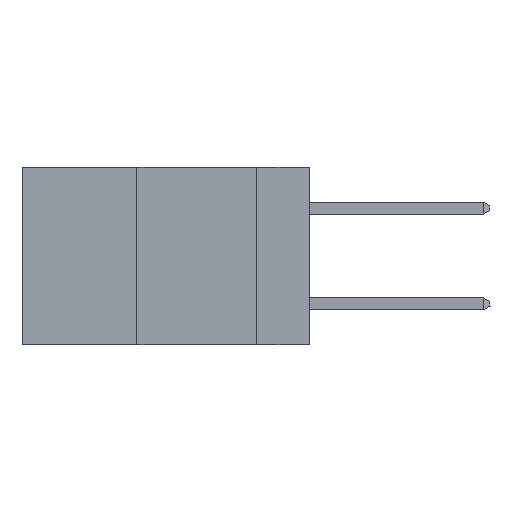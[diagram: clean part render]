
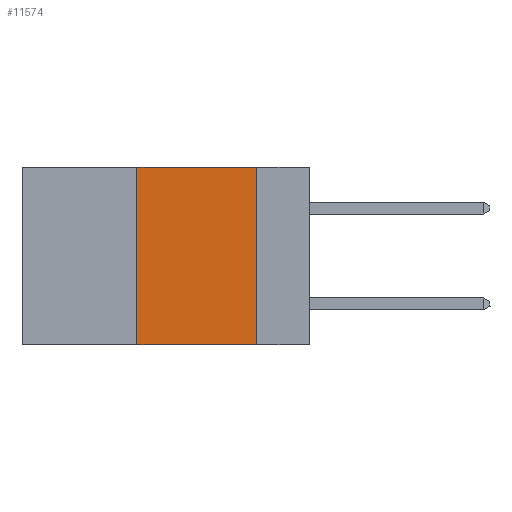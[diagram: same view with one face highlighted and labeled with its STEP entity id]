
A CAD part, left-side view. The second image highlights one B-rep face of the part: STEP entity #11574.
In plain terms, the highlighted planar face has unit normal (-1, 0, 0).
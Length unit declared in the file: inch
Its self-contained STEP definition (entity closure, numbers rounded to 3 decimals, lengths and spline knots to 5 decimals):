
#11 = CARTESIAN_POINT ( 'NONE',  ( 0., 0.11, 0. ) ) ;
#1041 = LINE ( 'NONE', #3717, #27874 ) ;
#1991 = LINE ( 'NONE', #10637, #17150 ) ;
#2290 = EDGE_CURVE ( 'NONE', #25126, #7796, #1991, .T. ) ;
#2810 = FACE_OUTER_BOUND ( 'NONE', #6803, .T. ) ;
#3507 = CARTESIAN_POINT ( 'NONE',  ( 0., 0.36, -0.37 ) ) ;
#3690 = CARTESIAN_POINT ( 'NONE',  ( 0., 0.6, 0. ) ) ;
#3717 = CARTESIAN_POINT ( 'NONE',  ( 0., 0.36, 0. ) ) ;
#4641 = ORIENTED_EDGE ( 'NONE', *, *, #2290, .F. ) ;
#5027 = EDGE_CURVE ( 'NONE', #16931, #7796, #6392, .T. ) ;
#5495 = VERTEX_POINT ( 'NONE', #27720 ) ;
#6392 = LINE ( 'NONE', #24162, #19843 ) ;
#6803 = EDGE_LOOP ( 'NONE', ( #4641, #9440, #10124, #21333 ) ) ;
#7796 = VERTEX_POINT ( 'NONE', #8721 ) ;
#8721 = CARTESIAN_POINT ( 'NONE',  ( 0., 0.11, -0.37 ) ) ;
#9440 = ORIENTED_EDGE ( 'NONE', *, *, #21893, .F. ) ;
#9798 = DIRECTION ( 'NONE',  ( 0., -1., 0. ) ) ;
#9995 = CARTESIAN_POINT ( 'NONE',  ( 0., 0.6, 0. ) ) ;
#10124 = ORIENTED_EDGE ( 'NONE', *, *, #17998, .F. ) ;
#10637 = CARTESIAN_POINT ( 'NONE',  ( 0., 0.11, 0. ) ) ;
#10648 = DIRECTION ( 'NONE',  ( 0., -1., 0. ) ) ;
#11574 = ADVANCED_FACE ( 'NONE', ( #2810 ), #17202, .F. ) ;
#13460 = VECTOR ( 'NONE', #9798, 39.37008 ) ;
#15278 = DIRECTION ( 'NONE',  ( 0., 0., -1. ) ) ;
#16931 = VERTEX_POINT ( 'NONE', #3507 ) ;
#17150 = VECTOR ( 'NONE', #15278, 39.37008 ) ;
#17202 = PLANE ( 'NONE',  #27908 ) ;
#17998 = EDGE_CURVE ( 'NONE', #16931, #5495, #1041, .T. ) ;
#19498 = DIRECTION ( 'NONE',  ( 0., 0., -1. ) ) ;
#19843 = VECTOR ( 'NONE', #10648, 39.37008 ) ;
#21333 = ORIENTED_EDGE ( 'NONE', *, *, #5027, .T. ) ;
#21893 = EDGE_CURVE ( 'NONE', #5495, #25126, #23345, .T. ) ;
#23345 = LINE ( 'NONE', #9995, #13460 ) ;
#24162 = CARTESIAN_POINT ( 'NONE',  ( 0., 0.6, -0.37 ) ) ;
#24431 = DIRECTION ( 'NONE',  ( 0., 0., 1. ) ) ;
#25126 = VERTEX_POINT ( 'NONE', #11 ) ;
#26482 = DIRECTION ( 'NONE',  ( 1., 0., 0. ) ) ;
#27720 = CARTESIAN_POINT ( 'NONE',  ( 0., 0.36, 0. ) ) ;
#27874 = VECTOR ( 'NONE', #24431, 39.37008 ) ;
#27908 = AXIS2_PLACEMENT_3D ( 'NONE', #3690, #26482, #19498 ) ;
